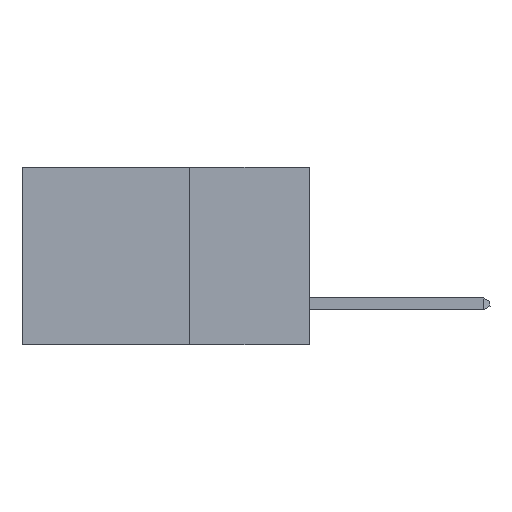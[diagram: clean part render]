
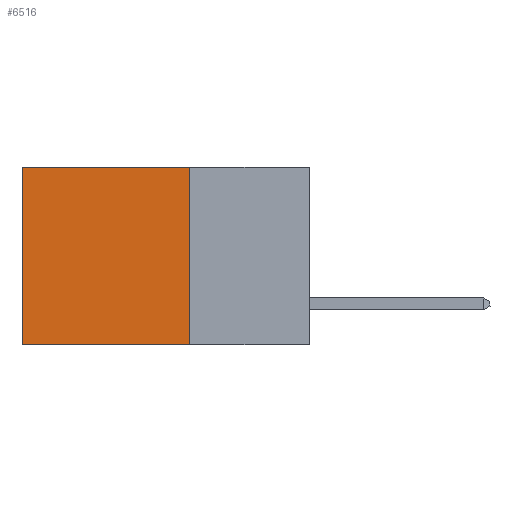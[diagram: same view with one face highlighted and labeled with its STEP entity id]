
A CAD part, left-side view. The second image highlights one B-rep face of the part: STEP entity #6516.
In plain terms, the highlighted planar face has unit normal (-1, 0, 0).
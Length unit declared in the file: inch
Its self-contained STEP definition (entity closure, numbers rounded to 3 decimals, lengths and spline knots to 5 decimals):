
#24 = FACE_OUTER_BOUND ( 'NONE', #23902, .T. ) ;
#61 = LINE ( 'NONE', #14413, #19990 ) ;
#1050 = DIRECTION ( 'NONE',  ( 0., 0., -1. ) ) ;
#2345 = EDGE_CURVE ( 'NONE', #14681, #10151, #15690, .T. ) ;
#2536 = CARTESIAN_POINT ( 'NONE',  ( 0.2875, 0.6, 0. ) ) ;
#4163 = EDGE_CURVE ( 'NONE', #18963, #24126, #14405, .T. ) ;
#4736 = DIRECTION ( 'NONE',  ( 0., 0., -1. ) ) ;
#6469 = DIRECTION ( 'NONE',  ( 0., 0., -1. ) ) ;
#6516 = ADVANCED_FACE ( 'NONE', ( #24 ), #10788, .F. ) ;
#8451 = ORIENTED_EDGE ( 'NONE', *, *, #4163, .F. ) ;
#8786 = EDGE_CURVE ( 'NONE', #10151, #24126, #23040, .T. ) ;
#10151 = VERTEX_POINT ( 'NONE', #12388 ) ;
#10553 = VECTOR ( 'NONE', #21994, 39.37008 ) ;
#10788 = PLANE ( 'NONE',  #24170 ) ;
#11383 = CARTESIAN_POINT ( 'NONE',  ( 0.2875, 0.6, -0.37 ) ) ;
#12107 = EDGE_CURVE ( 'NONE', #14681, #18963, #61, .T. ) ;
#12388 = CARTESIAN_POINT ( 'NONE',  ( 0.2875, 0.6, 0. ) ) ;
#12724 = DIRECTION ( 'NONE',  ( 1., 0., 0. ) ) ;
#14004 = CARTESIAN_POINT ( 'NONE',  ( 0.2875, 0.25, 0. ) ) ;
#14405 = LINE ( 'NONE', #18659, #24348 ) ;
#14413 = CARTESIAN_POINT ( 'NONE',  ( 0.2875, 0.25, 0. ) ) ;
#14681 = VERTEX_POINT ( 'NONE', #14004 ) ;
#15690 = LINE ( 'NONE', #24281, #10553 ) ;
#16548 = ORIENTED_EDGE ( 'NONE', *, *, #12107, .F. ) ;
#16997 = ORIENTED_EDGE ( 'NONE', *, *, #2345, .T. ) ;
#17755 = CARTESIAN_POINT ( 'NONE',  ( 0.2875, 0.25, -0.37 ) ) ;
#18659 = CARTESIAN_POINT ( 'NONE',  ( 0.2875, 0.25, -0.37 ) ) ;
#18963 = VERTEX_POINT ( 'NONE', #17755 ) ;
#19887 = DIRECTION ( 'NONE',  ( 0., 1., 0. ) ) ;
#19990 = VECTOR ( 'NONE', #4736, 39.37008 ) ;
#20648 = ORIENTED_EDGE ( 'NONE', *, *, #8786, .T. ) ;
#21994 = DIRECTION ( 'NONE',  ( 0., 1., 0. ) ) ;
#22458 = VECTOR ( 'NONE', #6469, 39.37008 ) ;
#23040 = LINE ( 'NONE', #2536, #22458 ) ;
#23902 = EDGE_LOOP ( 'NONE', ( #20648, #8451, #16548, #16997 ) ) ;
#23985 = CARTESIAN_POINT ( 'NONE',  ( 0.2875, 0.25, 0. ) ) ;
#24126 = VERTEX_POINT ( 'NONE', #11383 ) ;
#24170 = AXIS2_PLACEMENT_3D ( 'NONE', #23985, #12724, #1050 ) ;
#24281 = CARTESIAN_POINT ( 'NONE',  ( 0.2875, 0.25, 0. ) ) ;
#24348 = VECTOR ( 'NONE', #19887, 39.37008 ) ;
